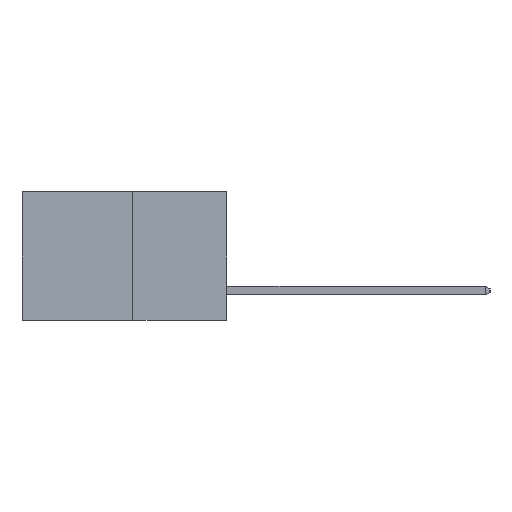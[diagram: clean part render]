
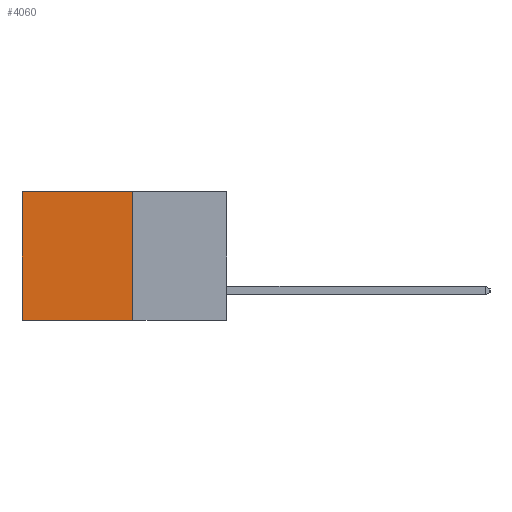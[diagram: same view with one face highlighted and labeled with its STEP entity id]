
A CAD part, left-side view. The second image highlights one B-rep face of the part: STEP entity #4060.
In plain terms, the highlighted planar face has unit normal (-1, 0, 0).
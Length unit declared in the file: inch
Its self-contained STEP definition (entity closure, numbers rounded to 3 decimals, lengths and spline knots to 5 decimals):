
#124 = PLANE ( 'NONE',  #6830 ) ;
#553 = EDGE_CURVE ( 'NONE', #5264, #9774, #9361, .T. ) ;
#603 = FACE_OUTER_BOUND ( 'NONE', #8281, .T. ) ;
#633 = ORIENTED_EDGE ( 'NONE', *, *, #553, .T. ) ;
#787 = CARTESIAN_POINT ( 'NONE',  ( 0.277, 0.59, 0. ) ) ;
#863 = DIRECTION ( 'NONE',  ( 0., 1., 0. ) ) ;
#1203 = VERTEX_POINT ( 'NONE', #6352 ) ;
#1470 = EDGE_CURVE ( 'NONE', #1203, #7933, #7609, .T. ) ;
#2316 = CARTESIAN_POINT ( 'NONE',  ( 0.277, 0.59, -0.37 ) ) ;
#2685 = CARTESIAN_POINT ( 'NONE',  ( 0.277, 0.27, -0.37 ) ) ;
#2704 = CARTESIAN_POINT ( 'NONE',  ( 0.277, 0.27, 0. ) ) ;
#2793 = DIRECTION ( 'NONE',  ( 0., 1., 0. ) ) ;
#3569 = VECTOR ( 'NONE', #6519, 39.37008 ) ;
#3598 = ORIENTED_EDGE ( 'NONE', *, *, #1470, .F. ) ;
#3711 = VECTOR ( 'NONE', #2793, 39.37008 ) ;
#4060 = ADVANCED_FACE ( 'NONE', ( #603 ), #124, .F. ) ;
#4258 = LINE ( 'NONE', #7233, #8126 ) ;
#5264 = VERTEX_POINT ( 'NONE', #9793 ) ;
#5576 = VECTOR ( 'NONE', #863, 39.37008 ) ;
#5703 = LINE ( 'NONE', #9482, #3569 ) ;
#6201 = EDGE_CURVE ( 'NONE', #9774, #7933, #4258, .T. ) ;
#6325 = DIRECTION ( 'NONE',  ( 0., 0., -1. ) ) ;
#6352 = CARTESIAN_POINT ( 'NONE',  ( 0.277, 0.27, -0.37 ) ) ;
#6356 = DIRECTION ( 'NONE',  ( 1., 0., 0. ) ) ;
#6519 = DIRECTION ( 'NONE',  ( 0., 0., -1. ) ) ;
#6830 = AXIS2_PLACEMENT_3D ( 'NONE', #2685, #6356, #6325 ) ;
#7233 = CARTESIAN_POINT ( 'NONE',  ( 0.277, 0.59, -0.37 ) ) ;
#7264 = DIRECTION ( 'NONE',  ( 0., 0., -1. ) ) ;
#7609 = LINE ( 'NONE', #9362, #5576 ) ;
#7933 = VERTEX_POINT ( 'NONE', #2316 ) ;
#8126 = VECTOR ( 'NONE', #7264, 39.37008 ) ;
#8127 = EDGE_CURVE ( 'NONE', #5264, #1203, #5703, .T. ) ;
#8281 = EDGE_LOOP ( 'NONE', ( #9488, #3598, #9692, #633 ) ) ;
#9361 = LINE ( 'NONE', #2704, #3711 ) ;
#9362 = CARTESIAN_POINT ( 'NONE',  ( 0.277, 0.27, -0.37 ) ) ;
#9482 = CARTESIAN_POINT ( 'NONE',  ( 0.277, 0.27, -0.37 ) ) ;
#9488 = ORIENTED_EDGE ( 'NONE', *, *, #6201, .T. ) ;
#9692 = ORIENTED_EDGE ( 'NONE', *, *, #8127, .F. ) ;
#9774 = VERTEX_POINT ( 'NONE', #787 ) ;
#9793 = CARTESIAN_POINT ( 'NONE',  ( 0.277, 0.27, 0. ) ) ;
